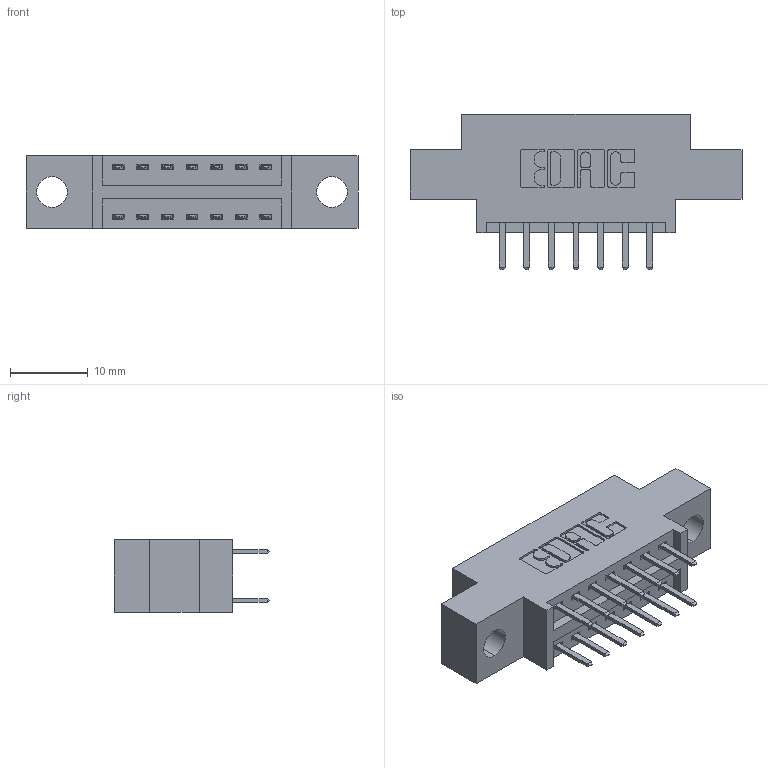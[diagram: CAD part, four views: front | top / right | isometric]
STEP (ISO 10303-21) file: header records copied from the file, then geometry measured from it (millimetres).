
FILE_DESCRIPTION (( 'STEP AP203' ), '1' );
FILE_NAME ('396-014-520-804.STEP', '2018-08-31T09:02:43', ( '' ), ( '' ), 'SwSTEP 2.0', 'SolidWorks 2016', '' );
FILE_SCHEMA (( 'CONFIG_CONTROL_DESIGN' ));
Length unit declared in the file: inch
Products named in the file (3): 346 Part_0.170 Offset - 0.156 Dia-TH; 345-292-001_345-293-120; 396-014-520-804
Assembly tree (15 placements, depth 2):
  396-014-520-804
    346 Part_0.170 Offset - 0.156 Dia-TH
    345-292-001_345-293-120  x14
Bounding box: 42.8 x 20.02 x 9.4 mm (x, y, z)
Volume: 3653 mm3; surface area: 4449.7 mm2
Topology: 15 solids, 15 shells, 910 faces, 2623 edges, 1710 vertices
Faces by surface type: plane 598, cylinder 312
Entity records: 9529 total; most frequent: CARTESIAN_POINT 1632, ORIENTED_EDGE 1554, DIRECTION 1477, EDGE_CURVE 777, LINE 613, VECTOR 613, VERTEX_POINT 514, AXIS2_PLACEMENT_3D 432
